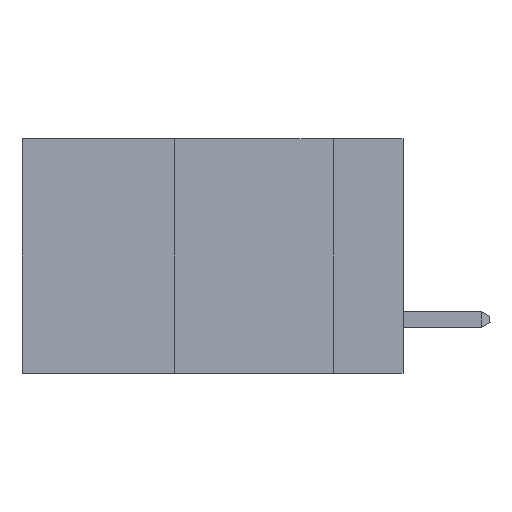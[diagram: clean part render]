
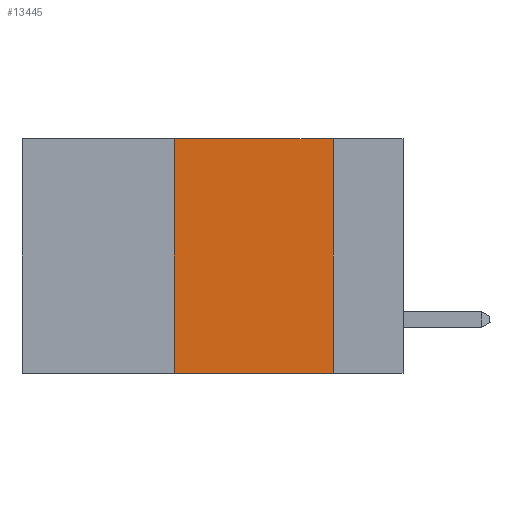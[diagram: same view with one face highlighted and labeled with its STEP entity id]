
A CAD part, left-side view. The second image highlights one B-rep face of the part: STEP entity #13445.
In plain terms, the highlighted planar face has unit normal (-1, 0, 0).
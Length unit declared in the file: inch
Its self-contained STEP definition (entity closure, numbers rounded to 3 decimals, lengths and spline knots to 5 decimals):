
#1183 = VERTEX_POINT ( 'NONE', #15933 ) ;
#1197 = DIRECTION ( 'NONE',  ( 0., 0., -1. ) ) ;
#2863 = ORIENTED_EDGE ( 'NONE', *, *, #12447, .F. ) ;
#2997 = PLANE ( 'NONE',  #14000 ) ;
#4183 = CARTESIAN_POINT ( 'NONE',  ( 0., 0.11, 0. ) ) ;
#5850 = FACE_OUTER_BOUND ( 'NONE', #11595, .T. ) ;
#5987 = VERTEX_POINT ( 'NONE', #7377 ) ;
#6777 = VECTOR ( 'NONE', #17337, 39.37008 ) ;
#6944 = DIRECTION ( 'NONE',  ( 0., -1., 0. ) ) ;
#7099 = VECTOR ( 'NONE', #1197, 39.37008 ) ;
#7377 = CARTESIAN_POINT ( 'NONE',  ( 0., 0.36, 0. ) ) ;
#7402 = CARTESIAN_POINT ( 'NONE',  ( 0., 0.6, 0. ) ) ;
#8327 = VECTOR ( 'NONE', #6944, 39.37008 ) ;
#8698 = DIRECTION ( 'NONE',  ( 0., -1., 0. ) ) ;
#8762 = CARTESIAN_POINT ( 'NONE',  ( 0., 0.11, 0. ) ) ;
#10167 = CARTESIAN_POINT ( 'NONE',  ( 0., 0.6, -0.37 ) ) ;
#10545 = ORIENTED_EDGE ( 'NONE', *, *, #11826, .F. ) ;
#11595 = EDGE_LOOP ( 'NONE', ( #12273, #10545, #2863, #16058 ) ) ;
#11826 = EDGE_CURVE ( 'NONE', #5987, #13036, #15518, .T. ) ;
#12273 = ORIENTED_EDGE ( 'NONE', *, *, #16940, .F. ) ;
#12447 = EDGE_CURVE ( 'NONE', #13636, #5987, #12483, .T. ) ;
#12483 = LINE ( 'NONE', #13130, #6777 ) ;
#12572 = CARTESIAN_POINT ( 'NONE',  ( 0., 0.6, 0. ) ) ;
#12727 = DIRECTION ( 'NONE',  ( 1., 0., 0. ) ) ;
#12962 = DIRECTION ( 'NONE',  ( 0., 0., -1. ) ) ;
#13018 = LINE ( 'NONE', #4183, #7099 ) ;
#13036 = VERTEX_POINT ( 'NONE', #8762 ) ;
#13130 = CARTESIAN_POINT ( 'NONE',  ( 0., 0.36, 0. ) ) ;
#13445 = ADVANCED_FACE ( 'NONE', ( #5850 ), #2997, .F. ) ;
#13486 = EDGE_CURVE ( 'NONE', #13636, #1183, #15271, .T. ) ;
#13636 = VERTEX_POINT ( 'NONE', #15878 ) ;
#14000 = AXIS2_PLACEMENT_3D ( 'NONE', #7402, #12727, #12962 ) ;
#14192 = VECTOR ( 'NONE', #8698, 39.37008 ) ;
#15271 = LINE ( 'NONE', #10167, #14192 ) ;
#15518 = LINE ( 'NONE', #12572, #8327 ) ;
#15878 = CARTESIAN_POINT ( 'NONE',  ( 0., 0.36, -0.37 ) ) ;
#15933 = CARTESIAN_POINT ( 'NONE',  ( 0., 0.11, -0.37 ) ) ;
#16058 = ORIENTED_EDGE ( 'NONE', *, *, #13486, .T. ) ;
#16940 = EDGE_CURVE ( 'NONE', #13036, #1183, #13018, .T. ) ;
#17337 = DIRECTION ( 'NONE',  ( 0., 0., 1. ) ) ;
